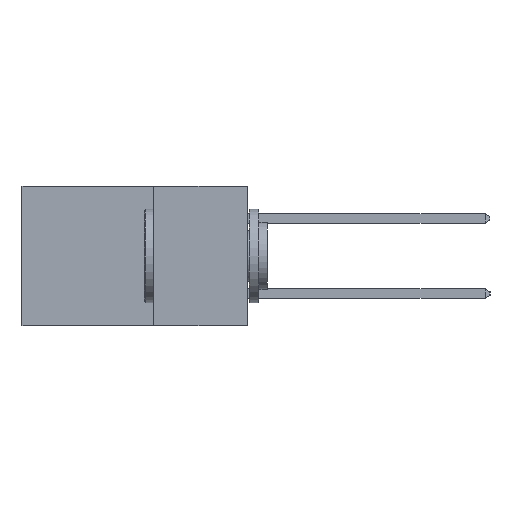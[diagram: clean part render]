
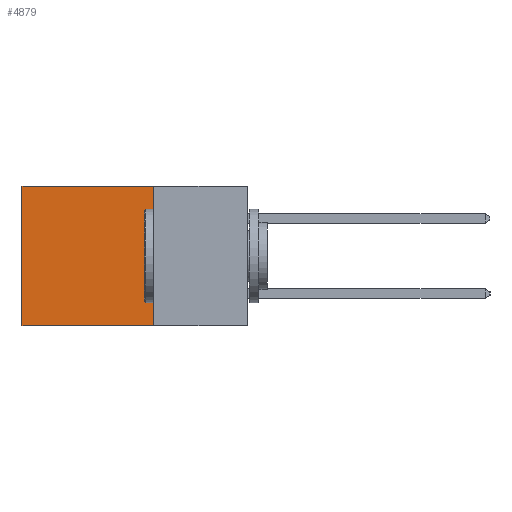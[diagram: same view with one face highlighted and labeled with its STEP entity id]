
A CAD part, left-side view. The second image highlights one B-rep face of the part: STEP entity #4879.
In plain terms, the highlighted planar face has unit normal (-1, 0, 0).
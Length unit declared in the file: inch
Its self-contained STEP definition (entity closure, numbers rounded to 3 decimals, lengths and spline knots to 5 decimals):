
#37 = CARTESIAN_POINT ( 'NONE',  ( 0.2615, 0.6, -0.37 ) ) ;
#199 = EDGE_LOOP ( 'NONE', ( #9938, #7813, #2469, #5417 ) ) ;
#471 = CARTESIAN_POINT ( 'NONE',  ( 0.2615, 0.25, 0. ) ) ;
#558 = DIRECTION ( 'NONE',  ( 0., 1., 0. ) ) ;
#1320 = VERTEX_POINT ( 'NONE', #1721 ) ;
#1417 = LINE ( 'NONE', #5887, #11697 ) ;
#1707 = CARTESIAN_POINT ( 'NONE',  ( 0.2615, 0.6, -0.37 ) ) ;
#1721 = CARTESIAN_POINT ( 'NONE',  ( 0.2615, 0.25, 0. ) ) ;
#1861 = DIRECTION ( 'NONE',  ( 0., 0., -1. ) ) ;
#2469 = ORIENTED_EDGE ( 'NONE', *, *, #6409, .F. ) ;
#3767 = DIRECTION ( 'NONE',  ( 0., 0., -1. ) ) ;
#3857 = DIRECTION ( 'NONE',  ( 1., 0., 0. ) ) ;
#4134 = AXIS2_PLACEMENT_3D ( 'NONE', #4287, #3857, #3767 ) ;
#4287 = CARTESIAN_POINT ( 'NONE',  ( 0.2615, 0.25, -0.37 ) ) ;
#4429 = PLANE ( 'NONE',  #4134 ) ;
#4879 = ADVANCED_FACE ( 'NONE', ( #9919 ), #4429, .F. ) ;
#5123 = VECTOR ( 'NONE', #558, 39.37008 ) ;
#5174 = VERTEX_POINT ( 'NONE', #37 ) ;
#5417 = ORIENTED_EDGE ( 'NONE', *, *, #5761, .T. ) ;
#5471 = EDGE_CURVE ( 'NONE', #5889, #5174, #6331, .T. ) ;
#5558 = VECTOR ( 'NONE', #8658, 39.37008 ) ;
#5761 = EDGE_CURVE ( 'NONE', #1320, #5889, #10405, .T. ) ;
#5860 = DIRECTION ( 'NONE',  ( 0., 1., 0. ) ) ;
#5887 = CARTESIAN_POINT ( 'NONE',  ( 0.2615, 0.25, -0.37 ) ) ;
#5889 = VERTEX_POINT ( 'NONE', #10567 ) ;
#6331 = LINE ( 'NONE', #1707, #8674 ) ;
#6409 = EDGE_CURVE ( 'NONE', #1320, #10358, #8204, .T. ) ;
#7813 = ORIENTED_EDGE ( 'NONE', *, *, #7848, .F. ) ;
#7848 = EDGE_CURVE ( 'NONE', #10358, #5174, #1417, .T. ) ;
#8204 = LINE ( 'NONE', #8685, #5558 ) ;
#8658 = DIRECTION ( 'NONE',  ( 0., 0., -1. ) ) ;
#8674 = VECTOR ( 'NONE', #1861, 39.37008 ) ;
#8685 = CARTESIAN_POINT ( 'NONE',  ( 0.2615, 0.25, -0.37 ) ) ;
#9919 = FACE_OUTER_BOUND ( 'NONE', #199, .T. ) ;
#9938 = ORIENTED_EDGE ( 'NONE', *, *, #5471, .T. ) ;
#10358 = VERTEX_POINT ( 'NONE', #11675 ) ;
#10405 = LINE ( 'NONE', #471, #5123 ) ;
#10567 = CARTESIAN_POINT ( 'NONE',  ( 0.2615, 0.6, 0. ) ) ;
#11675 = CARTESIAN_POINT ( 'NONE',  ( 0.2615, 0.25, -0.37 ) ) ;
#11697 = VECTOR ( 'NONE', #5860, 39.37008 ) ;
